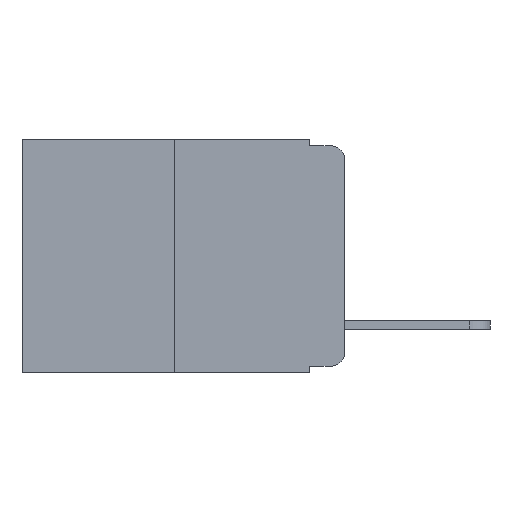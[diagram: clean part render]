
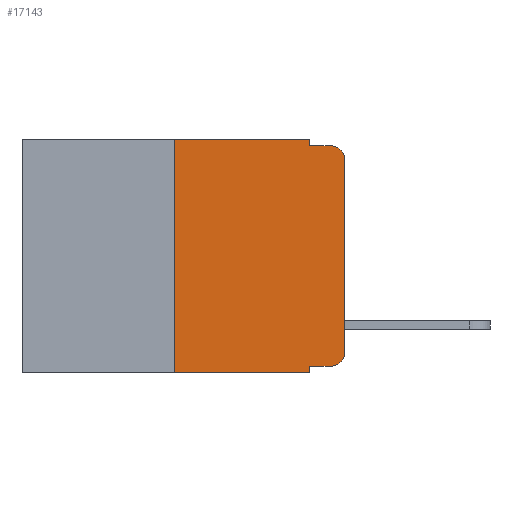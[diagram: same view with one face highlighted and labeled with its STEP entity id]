
A CAD part, left-side view. The second image highlights one B-rep face of the part: STEP entity #17143.
In plain terms, the highlighted planar face has unit normal (-1, 0, 0).
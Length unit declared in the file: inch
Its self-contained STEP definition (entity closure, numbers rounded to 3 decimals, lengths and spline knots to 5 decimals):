
#73 = CARTESIAN_POINT ( 'NONE',  ( 0., 0.25, -0.343 ) ) ;
#215 = ORIENTED_EDGE ( 'NONE', *, *, #1332, .T. ) ;
#487 = VECTOR ( 'NONE', #5659, 39.37008 ) ;
#568 = VECTOR ( 'NONE', #17052, 39.37008 ) ;
#668 = EDGE_CURVE ( 'NONE', #14879, #14774, #14217, .T. ) ;
#1132 = LINE ( 'NONE', #17543, #568 ) ;
#1212 = CARTESIAN_POINT ( 'NONE',  ( 0., 0.25, 0. ) ) ;
#1279 = LINE ( 'NONE', #19005, #5654 ) ;
#1327 = EDGE_CURVE ( 'NONE', #20873, #12332, #4188, .T. ) ;
#1332 = EDGE_CURVE ( 'NONE', #12332, #6636, #12725, .T. ) ;
#1356 = EDGE_CURVE ( 'NONE', #21849, #6636, #3553, .T. ) ;
#1362 = EDGE_CURVE ( 'NONE', #14278, #21849, #2982, .T. ) ;
#1396 = EDGE_CURVE ( 'NONE', #14879, #14817, #15468, .T. ) ;
#1397 = EDGE_CURVE ( 'NONE', #8519, #14774, #6710, .T. ) ;
#1428 = EDGE_CURVE ( 'NONE', #8519, #6586, #1279, .T. ) ;
#1433 = EDGE_CURVE ( 'NONE', #6586, #20873, #10681, .T. ) ;
#1844 = VECTOR ( 'NONE', #9561, 39.37008 ) ;
#2041 = CARTESIAN_POINT ( 'NONE',  ( 0., 0.02, -0.333 ) ) ;
#2328 = CARTESIAN_POINT ( 'NONE',  ( 0., 0.051, -0.343 ) ) ;
#2982 = LINE ( 'NONE', #11835, #11717 ) ;
#3079 = CARTESIAN_POINT ( 'NONE',  ( 0., 0.051, -0.333 ) ) ;
#3553 = LINE ( 'NONE', #14889, #20777 ) ;
#4050 = PLANE ( 'NONE',  #17993 ) ;
#4188 = LINE ( 'NONE', #6375, #17051 ) ;
#4307 = CARTESIAN_POINT ( 'NONE',  ( 0., 0.473, -0.343 ) ) ;
#4403 = EDGE_CURVE ( 'NONE', #14817, #14278, #1132, .T. ) ;
#4892 = CARTESIAN_POINT ( 'NONE',  ( 0., 0., -0.313 ) ) ;
#5162 = ORIENTED_EDGE ( 'NONE', *, *, #1356, .F. ) ;
#5654 = VECTOR ( 'NONE', #18345, 39.37008 ) ;
#5659 = DIRECTION ( 'NONE',  ( 0., -1., 0. ) ) ;
#6375 = CARTESIAN_POINT ( 'NONE',  ( 0., 0., 0. ) ) ;
#6586 = VERTEX_POINT ( 'NONE', #2041 ) ;
#6636 = VERTEX_POINT ( 'NONE', #21371 ) ;
#6710 = LINE ( 'NONE', #12200, #14929 ) ;
#7370 = ORIENTED_EDGE ( 'NONE', *, *, #1428, .T. ) ;
#7605 = DIRECTION ( 'NONE',  ( 0., 0., -1. ) ) ;
#7636 = ORIENTED_EDGE ( 'NONE', *, *, #4403, .F. ) ;
#7670 = DIRECTION ( 'NONE',  ( 1., 0., 0. ) ) ;
#8186 = ORIENTED_EDGE ( 'NONE', *, *, #1396, .F. ) ;
#8519 = VERTEX_POINT ( 'NONE', #3079 ) ;
#9561 = DIRECTION ( 'NONE',  ( 0., 0., 1. ) ) ;
#10043 = CARTESIAN_POINT ( 'NONE',  ( 0., 0.051, -0.01 ) ) ;
#10681 = CIRCLE ( 'NONE', #14363, 0.02 ) ;
#10777 = ORIENTED_EDGE ( 'NONE', *, *, #1397, .F. ) ;
#11189 = AXIS2_PLACEMENT_3D ( 'NONE', #14868, #14836, #12628 ) ;
#11717 = VECTOR ( 'NONE', #7605, 39.37008 ) ;
#11766 = DIRECTION ( 'NONE',  ( 0., 0., 1. ) ) ;
#11835 = CARTESIAN_POINT ( 'NONE',  ( 0., 0.051, 0. ) ) ;
#12200 = CARTESIAN_POINT ( 'NONE',  ( 0., 0.051, 0. ) ) ;
#12287 = CARTESIAN_POINT ( 'NONE',  ( 0., 0.051, 0. ) ) ;
#12332 = VERTEX_POINT ( 'NONE', #18560 ) ;
#12547 = ORIENTED_EDGE ( 'NONE', *, *, #668, .T. ) ;
#12628 = DIRECTION ( 'NONE',  ( 0., 0., -1. ) ) ;
#12725 = CIRCLE ( 'NONE', #11189, 0.02 ) ;
#13457 = DIRECTION ( 'NONE',  ( 0., 0., -1. ) ) ;
#14217 = LINE ( 'NONE', #4307, #487 ) ;
#14278 = VERTEX_POINT ( 'NONE', #12287 ) ;
#14363 = AXIS2_PLACEMENT_3D ( 'NONE', #17418, #17346, #16791 ) ;
#14774 = VERTEX_POINT ( 'NONE', #2328 ) ;
#14817 = VERTEX_POINT ( 'NONE', #1212 ) ;
#14836 = DIRECTION ( 'NONE',  ( -1., 0., 0. ) ) ;
#14868 = CARTESIAN_POINT ( 'NONE',  ( 0., 0.02, -0.03 ) ) ;
#14879 = VERTEX_POINT ( 'NONE', #73 ) ;
#14889 = CARTESIAN_POINT ( 'NONE',  ( 0., 0.051, -0.01 ) ) ;
#14929 = VECTOR ( 'NONE', #13457, 39.37008 ) ;
#15042 = CARTESIAN_POINT ( 'NONE',  ( 0., 0.25, 0. ) ) ;
#15468 = LINE ( 'NONE', #15042, #1844 ) ;
#15707 = DIRECTION ( 'NONE',  ( 0., -1., 0. ) ) ;
#16328 = ORIENTED_EDGE ( 'NONE', *, *, #1327, .T. ) ;
#16791 = DIRECTION ( 'NONE',  ( 0., 0., -1. ) ) ;
#17051 = VECTOR ( 'NONE', #11766, 39.37008 ) ;
#17052 = DIRECTION ( 'NONE',  ( 0., -1., 0. ) ) ;
#17143 = ADVANCED_FACE ( 'NONE', ( #17821 ), #4050, .F. ) ;
#17346 = DIRECTION ( 'NONE',  ( -1., 0., 0. ) ) ;
#17418 = CARTESIAN_POINT ( 'NONE',  ( 0., 0.02, -0.313 ) ) ;
#17543 = CARTESIAN_POINT ( 'NONE',  ( 0., 0.473, 0. ) ) ;
#17821 = FACE_OUTER_BOUND ( 'NONE', #19341, .T. ) ;
#17993 = AXIS2_PLACEMENT_3D ( 'NONE', #20602, #7670, #19141 ) ;
#18345 = DIRECTION ( 'NONE',  ( 0., -1., 0. ) ) ;
#18560 = CARTESIAN_POINT ( 'NONE',  ( 0., 0., -0.03 ) ) ;
#18905 = ORIENTED_EDGE ( 'NONE', *, *, #1362, .F. ) ;
#19005 = CARTESIAN_POINT ( 'NONE',  ( 0., 0.051, -0.333 ) ) ;
#19141 = DIRECTION ( 'NONE',  ( 0., 0., -1. ) ) ;
#19341 = EDGE_LOOP ( 'NONE', ( #16328, #215, #5162, #18905, #7636, #8186, #12547, #10777, #7370, #20871 ) ) ;
#20602 = CARTESIAN_POINT ( 'NONE',  ( 0., 0.473, 0. ) ) ;
#20777 = VECTOR ( 'NONE', #15707, 39.37008 ) ;
#20871 = ORIENTED_EDGE ( 'NONE', *, *, #1433, .T. ) ;
#20873 = VERTEX_POINT ( 'NONE', #4892 ) ;
#21371 = CARTESIAN_POINT ( 'NONE',  ( 0., 0.02, -0.01 ) ) ;
#21849 = VERTEX_POINT ( 'NONE', #10043 ) ;
